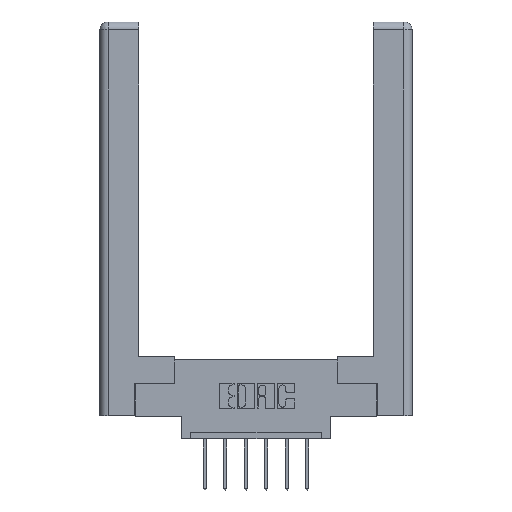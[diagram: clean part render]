
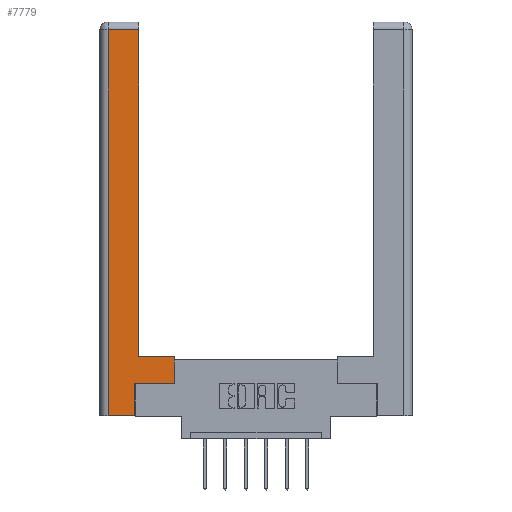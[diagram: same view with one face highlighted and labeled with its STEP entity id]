
A CAD part, top view. The second image highlights one B-rep face of the part: STEP entity #7779.
In plain terms, the highlighted planar face has unit normal (0, 0, 1).
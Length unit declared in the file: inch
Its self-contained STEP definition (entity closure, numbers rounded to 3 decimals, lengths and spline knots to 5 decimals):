
#181 = VERTEX_POINT ( 'NONE', #4587 ) ;
#273 = FACE_OUTER_BOUND ( 'NONE', #3573, .T. ) ;
#315 = VERTEX_POINT ( 'NONE', #8867 ) ;
#351 = PLANE ( 'NONE',  #6868 ) ;
#708 = ORIENTED_EDGE ( 'NONE', *, *, #11233, .T. ) ;
#725 = LINE ( 'NONE', #1327, #4872 ) ;
#760 = LINE ( 'NONE', #1445, #5183 ) ;
#822 = EDGE_CURVE ( 'NONE', #181, #1716, #725, .T. ) ;
#1054 = LINE ( 'NONE', #1057, #5320 ) ;
#1057 = CARTESIAN_POINT ( 'NONE',  ( 0.295, 3., 0. ) ) ;
#1186 = ORIENTED_EDGE ( 'NONE', *, *, #3788, .T. ) ;
#1327 = CARTESIAN_POINT ( 'NONE',  ( 0.0615, 2.94, 0. ) ) ;
#1445 = CARTESIAN_POINT ( 'NONE',  ( 0.295, 0.45, 0. ) ) ;
#1716 = VERTEX_POINT ( 'NONE', #6668 ) ;
#1820 = LINE ( 'NONE', #10325, #6421 ) ;
#1985 = DIRECTION ( 'NONE',  ( 1., 0., 0. ) ) ;
#2045 = CARTESIAN_POINT ( 'NONE',  ( 0., 0., 0. ) ) ;
#2121 = ORIENTED_EDGE ( 'NONE', *, *, #822, .T. ) ;
#2753 = VECTOR ( 'NONE', #5572, 39.37008 ) ;
#3017 = DIRECTION ( 'NONE',  ( 0., 0., -1. ) ) ;
#3573 = EDGE_LOOP ( 'NONE', ( #10305, #2121, #1186, #4938, #5940, #8482, #4214, #708 ) ) ;
#3788 = EDGE_CURVE ( 'NONE', #1716, #4468, #5954, .T. ) ;
#3913 = CARTESIAN_POINT ( 'NONE',  ( 0.265, 0.245, 0. ) ) ;
#4214 = ORIENTED_EDGE ( 'NONE', *, *, #4286, .T. ) ;
#4286 = EDGE_CURVE ( 'NONE', #9715, #6741, #6489, .T. ) ;
#4405 = CARTESIAN_POINT ( 'NONE',  ( 0.0615, 0., 0. ) ) ;
#4468 = VERTEX_POINT ( 'NONE', #4405 ) ;
#4587 = CARTESIAN_POINT ( 'NONE',  ( 0.295, 2.94, 0. ) ) ;
#4650 = DIRECTION ( 'NONE',  ( 0., 1., 0. ) ) ;
#4724 = VECTOR ( 'NONE', #4736, 39.37008 ) ;
#4736 = DIRECTION ( 'NONE',  ( 0., 1., 0. ) ) ;
#4872 = VECTOR ( 'NONE', #8658, 39.37008 ) ;
#4938 = ORIENTED_EDGE ( 'NONE', *, *, #7287, .T. ) ;
#5037 = DIRECTION ( 'NONE',  ( -1., 0., 0. ) ) ;
#5183 = VECTOR ( 'NONE', #5037, 39.37008 ) ;
#5219 = VECTOR ( 'NONE', #6207, 39.37008 ) ;
#5320 = VECTOR ( 'NONE', #4650, 39.37008 ) ;
#5572 = DIRECTION ( 'NONE',  ( 1., 0., 0. ) ) ;
#5655 = CARTESIAN_POINT ( 'NONE',  ( 0.565, 0.245, 0. ) ) ;
#5671 = DIRECTION ( 'NONE',  ( -1., 0., 0. ) ) ;
#5830 = EDGE_CURVE ( 'NONE', #315, #181, #1054, .T. ) ;
#5940 = ORIENTED_EDGE ( 'NONE', *, *, #6589, .T. ) ;
#5954 = LINE ( 'NONE', #10811, #5219 ) ;
#6207 = DIRECTION ( 'NONE',  ( 0., -1., 0. ) ) ;
#6421 = VECTOR ( 'NONE', #1985, 39.37008 ) ;
#6489 = LINE ( 'NONE', #11526, #9232 ) ;
#6589 = EDGE_CURVE ( 'NONE', #9912, #8251, #6997, .T. ) ;
#6624 = CARTESIAN_POINT ( 'NONE',  ( 0.565, 0.245, 0. ) ) ;
#6668 = CARTESIAN_POINT ( 'NONE',  ( 0.0615, 2.94, 0. ) ) ;
#6741 = VERTEX_POINT ( 'NONE', #7718 ) ;
#6788 = CARTESIAN_POINT ( 'NONE',  ( 0.265, 0., 0. ) ) ;
#6868 = AXIS2_PLACEMENT_3D ( 'NONE', #2045, #3017, #5671 ) ;
#6997 = LINE ( 'NONE', #9275, #4724 ) ;
#7045 = LINE ( 'NONE', #5655, #2753 ) ;
#7287 = EDGE_CURVE ( 'NONE', #4468, #9912, #1820, .T. ) ;
#7718 = CARTESIAN_POINT ( 'NONE',  ( 0.565, 0.45, 0. ) ) ;
#7779 = ADVANCED_FACE ( 'NONE', ( #273 ), #351, .F. ) ;
#8251 = VERTEX_POINT ( 'NONE', #3913 ) ;
#8482 = ORIENTED_EDGE ( 'NONE', *, *, #10906, .T. ) ;
#8658 = DIRECTION ( 'NONE',  ( -1., 0., 0. ) ) ;
#8662 = DIRECTION ( 'NONE',  ( 0., 1., 0. ) ) ;
#8867 = CARTESIAN_POINT ( 'NONE',  ( 0.295, 0.45, 0. ) ) ;
#9232 = VECTOR ( 'NONE', #8662, 39.37008 ) ;
#9275 = CARTESIAN_POINT ( 'NONE',  ( 0.265, 0.245, 0. ) ) ;
#9715 = VERTEX_POINT ( 'NONE', #6624 ) ;
#9912 = VERTEX_POINT ( 'NONE', #6788 ) ;
#10305 = ORIENTED_EDGE ( 'NONE', *, *, #5830, .T. ) ;
#10325 = CARTESIAN_POINT ( 'NONE',  ( 0.265, 0., 0. ) ) ;
#10811 = CARTESIAN_POINT ( 'NONE',  ( 0.0615, 0., 0. ) ) ;
#10906 = EDGE_CURVE ( 'NONE', #8251, #9715, #7045, .T. ) ;
#11233 = EDGE_CURVE ( 'NONE', #6741, #315, #760, .T. ) ;
#11526 = CARTESIAN_POINT ( 'NONE',  ( 0.565, 0.45, 0. ) ) ;
